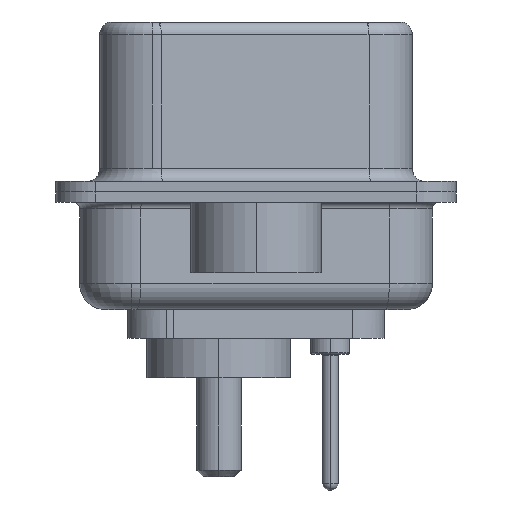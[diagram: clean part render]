
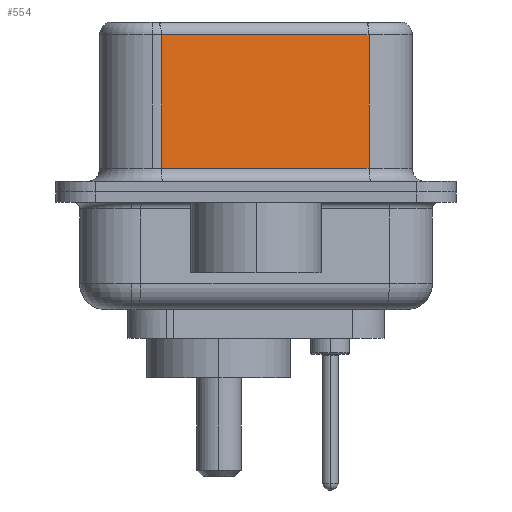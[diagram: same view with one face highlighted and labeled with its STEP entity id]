
A CAD part, left-side view. The second image highlights one B-rep face of the part: STEP entity #554.
In plain terms, the highlighted planar face has unit normal (-0.985, -0.174, 0).
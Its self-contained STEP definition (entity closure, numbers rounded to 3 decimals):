
#18 = VERTEX_POINT ( 'NONE', #14405 ) ;
#481 = DIRECTION ( 'NONE',  ( 0., 0., -1. ) ) ;
#554 = ADVANCED_FACE ( 'NONE', ( #21175 ), #1557, .F. ) ;
#616 = VECTOR ( 'NONE', #9634, 1000. ) ;
#950 = CARTESIAN_POINT ( 'NONE',  ( 5.132, -4.322, 0.9 ) ) ;
#1148 = EDGE_CURVE ( 'NONE', #8730, #1349, #10933, .T. ) ;
#1349 = VERTEX_POINT ( 'NONE', #13543 ) ;
#1557 = PLANE ( 'NONE',  #10859 ) ;
#2048 = DIRECTION ( 'NONE',  ( 0.985, 0.174, 0. ) ) ;
#2789 = EDGE_CURVE ( 'NONE', #18, #1349, #18026, .T. ) ;
#3852 = ORIENTED_EDGE ( 'NONE', *, *, #1148, .T. ) ;
#4568 = VERTEX_POINT ( 'NONE', #15382 ) ;
#4638 = DIRECTION ( 'NONE',  ( -0.174, 0.985, 0. ) ) ;
#5942 = CARTESIAN_POINT ( 'NONE',  ( 3.73, 3.628, 0.9 ) ) ;
#6033 = CARTESIAN_POINT ( 'NONE',  ( 5.132, -4.322, 6.52 ) ) ;
#6301 = EDGE_LOOP ( 'NONE', ( #16837, #10121, #16047, #3852 ) ) ;
#6547 = VECTOR ( 'NONE', #481, 1000. ) ;
#6939 = DIRECTION ( 'NONE',  ( -0.174, 0.985, 0. ) ) ;
#8730 = VERTEX_POINT ( 'NONE', #5942 ) ;
#9443 = CARTESIAN_POINT ( 'NONE',  ( 5.132, -4.322, 6.02 ) ) ;
#9634 = DIRECTION ( 'NONE',  ( 0., 0., -1. ) ) ;
#10121 = ORIENTED_EDGE ( 'NONE', *, *, #16729, .T. ) ;
#10491 = EDGE_CURVE ( 'NONE', #4568, #8730, #19584, .T. ) ;
#10735 = CARTESIAN_POINT ( 'NONE',  ( 5.132, -4.322, 6.52 ) ) ;
#10859 = AXIS2_PLACEMENT_3D ( 'NONE', #10735, #2048, #6939 ) ;
#10933 = LINE ( 'NONE', #950, #19086 ) ;
#13073 = DIRECTION ( 'NONE',  ( 0.174, -0.985, 0. ) ) ;
#13543 = CARTESIAN_POINT ( 'NONE',  ( 5.132, -4.322, 0.9 ) ) ;
#14405 = CARTESIAN_POINT ( 'NONE',  ( 5.132, -4.322, 6.02 ) ) ;
#15382 = CARTESIAN_POINT ( 'NONE',  ( 3.73, 3.628, 6.02 ) ) ;
#16047 = ORIENTED_EDGE ( 'NONE', *, *, #10491, .T. ) ;
#16664 = VECTOR ( 'NONE', #4638, 1000. ) ;
#16729 = EDGE_CURVE ( 'NONE', #18, #4568, #20995, .T. ) ;
#16837 = ORIENTED_EDGE ( 'NONE', *, *, #2789, .F. ) ;
#18026 = LINE ( 'NONE', #6033, #616 ) ;
#19086 = VECTOR ( 'NONE', #13073, 1000. ) ;
#19584 = LINE ( 'NONE', #20091, #6547 ) ;
#20091 = CARTESIAN_POINT ( 'NONE',  ( 3.73, 3.628, 6.52 ) ) ;
#20995 = LINE ( 'NONE', #9443, #16664 ) ;
#21175 = FACE_OUTER_BOUND ( 'NONE', #6301, .T. ) ;
